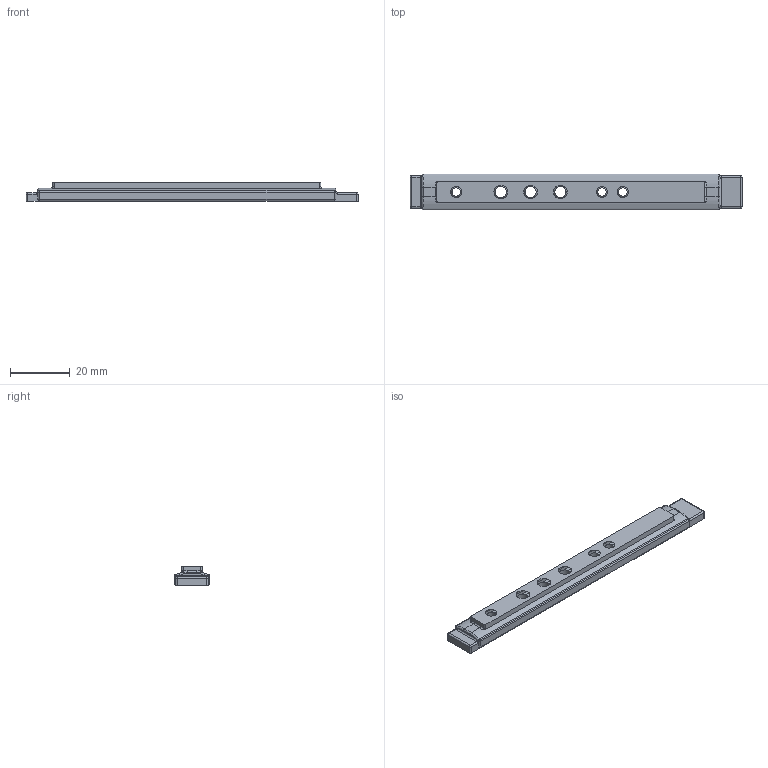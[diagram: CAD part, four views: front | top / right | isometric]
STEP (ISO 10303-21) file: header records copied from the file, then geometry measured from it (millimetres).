
FILE_DESCRIPTION(/* description */ (''),/* implementation_level */ '2;1');
FILE_NAME(/* name */ 'ARK Chargin'' Handle/Slide.step',/* time_stamp */ '2022-02-02T21:15:37-07:00',/* author */ (''),/* organization */ (''),/* preprocessor_version */ 'ST-DEVELOPER v18.1',/* originating_system */ 'Autodesk Translation Framework v10.13.0.1454',/* authorisation */ '');
FILE_SCHEMA (('AUTOMOTIVE_DESIGN { 1 0 10303 214 3 1 1 }'));
Length unit declared in the file: millimetre
Products named in the file (2): Jelly's ARK 2; GuidedHandle
Assembly tree (1 placements, depth 2):
  Jelly's ARK 2
    GuidedHandle
Bounding box: 111.5 x 12 x 6.35 mm (x, y, z)
Volume: 6262.4 mm3; surface area: 4083.6 mm2
Topology: 1 solids, 1 shells, 106 faces, 254 edges, 146 vertices
Faces by surface type: cylinder 38, plane 24, cone 16, bspline 12, sphere 8, torus 8
Full cylindrical faces by diameter (mm): 2.8 x3, 3.8 x3
Entity records: 3574 total; most frequent: CARTESIAN_POINT 1099, DIRECTION 506, ORIENTED_EDGE 500, EDGE_CURVE 250, AXIS2_PLACEMENT_3D 201, VERTEX_POINT 146, EDGE_LOOP 118, FACE_OUTER_BOUND 106
